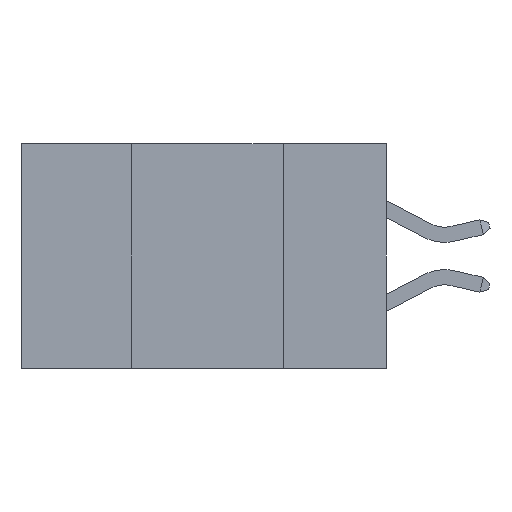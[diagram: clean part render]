
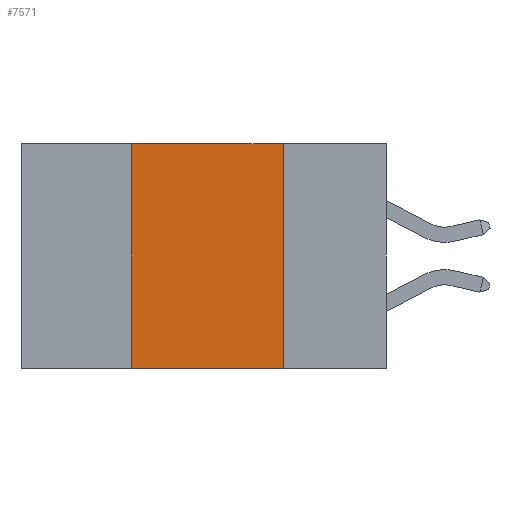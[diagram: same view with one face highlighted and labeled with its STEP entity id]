
A CAD part, left-side view. The second image highlights one B-rep face of the part: STEP entity #7571.
In plain terms, the highlighted planar face has unit normal (-1, 0, 0).
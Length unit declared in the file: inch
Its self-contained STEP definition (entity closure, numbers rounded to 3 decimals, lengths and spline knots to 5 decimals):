
#963 = CARTESIAN_POINT ( 'NONE',  ( 0., 0.17, -0.37 ) ) ;
#1656 = LINE ( 'NONE', #8428, #5064 ) ;
#1859 = VECTOR ( 'NONE', #11011, 39.37008 ) ;
#2236 = VECTOR ( 'NONE', #9684, 39.37008 ) ;
#2256 = EDGE_CURVE ( 'NONE', #2798, #2914, #1656, .T. ) ;
#2448 = DIRECTION ( 'NONE',  ( 0., 0., -1. ) ) ;
#2453 = CARTESIAN_POINT ( 'NONE',  ( 0., 0.6, -0.37 ) ) ;
#2629 = CARTESIAN_POINT ( 'NONE',  ( 0., 0.42, -0.37 ) ) ;
#2798 = VERTEX_POINT ( 'NONE', #11236 ) ;
#2914 = VERTEX_POINT ( 'NONE', #963 ) ;
#2997 = CARTESIAN_POINT ( 'NONE',  ( 0., 0.42, 0. ) ) ;
#3506 = FACE_OUTER_BOUND ( 'NONE', #7039, .T. ) ;
#4257 = LINE ( 'NONE', #4819, #2236 ) ;
#4490 = PLANE ( 'NONE',  #11293 ) ;
#4819 = CARTESIAN_POINT ( 'NONE',  ( 0., 0.6, 0. ) ) ;
#5064 = VECTOR ( 'NONE', #11138, 39.37008 ) ;
#6546 = EDGE_CURVE ( 'NONE', #6861, #2798, #4257, .T. ) ;
#6685 = CARTESIAN_POINT ( 'NONE',  ( 0., 0.42, -0.37 ) ) ;
#6861 = VERTEX_POINT ( 'NONE', #2997 ) ;
#7039 = EDGE_LOOP ( 'NONE', ( #11862, #9284, #8493, #8552 ) ) ;
#7277 = CARTESIAN_POINT ( 'NONE',  ( 0., 0.6, 0. ) ) ;
#7571 = ADVANCED_FACE ( 'NONE', ( #3506 ), #4490, .F. ) ;
#8013 = DIRECTION ( 'NONE',  ( 1., 0., 0. ) ) ;
#8067 = LINE ( 'NONE', #2453, #1859 ) ;
#8121 = LINE ( 'NONE', #2629, #11886 ) ;
#8191 = DIRECTION ( 'NONE',  ( 0., 0., 1. ) ) ;
#8428 = CARTESIAN_POINT ( 'NONE',  ( 0., 0.17, -0.37 ) ) ;
#8493 = ORIENTED_EDGE ( 'NONE', *, *, #8955, .F. ) ;
#8552 = ORIENTED_EDGE ( 'NONE', *, *, #8910, .T. ) ;
#8910 = EDGE_CURVE ( 'NONE', #10791, #2914, #8067, .T. ) ;
#8955 = EDGE_CURVE ( 'NONE', #10791, #6861, #8121, .T. ) ;
#9284 = ORIENTED_EDGE ( 'NONE', *, *, #6546, .F. ) ;
#9684 = DIRECTION ( 'NONE',  ( 0., -1., 0. ) ) ;
#10791 = VERTEX_POINT ( 'NONE', #6685 ) ;
#11011 = DIRECTION ( 'NONE',  ( 0., -1., 0. ) ) ;
#11138 = DIRECTION ( 'NONE',  ( 0., 0., -1. ) ) ;
#11236 = CARTESIAN_POINT ( 'NONE',  ( 0., 0.17, 0. ) ) ;
#11293 = AXIS2_PLACEMENT_3D ( 'NONE', #7277, #8013, #2448 ) ;
#11862 = ORIENTED_EDGE ( 'NONE', *, *, #2256, .F. ) ;
#11886 = VECTOR ( 'NONE', #8191, 39.37008 ) ;
